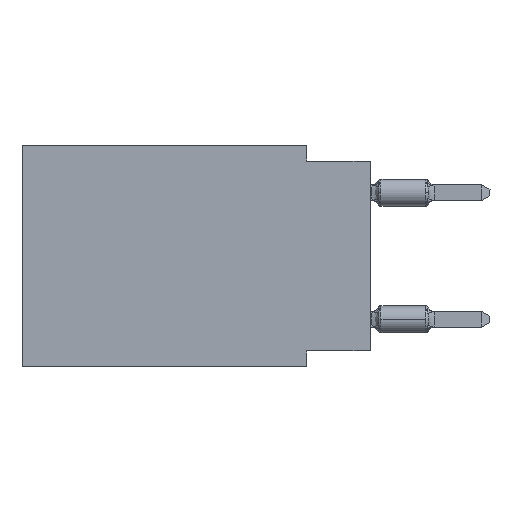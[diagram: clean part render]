
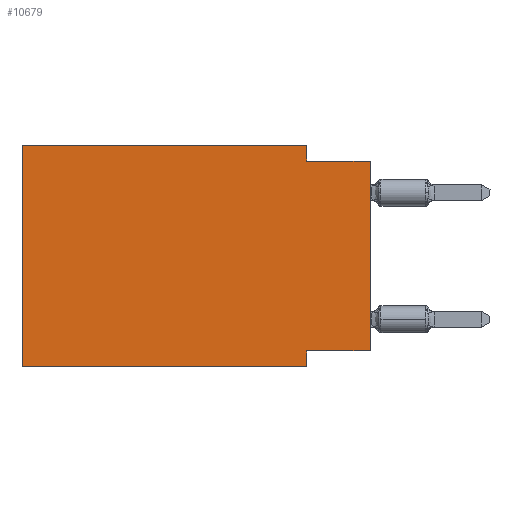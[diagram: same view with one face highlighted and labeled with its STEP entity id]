
A CAD part, left-side view. The second image highlights one B-rep face of the part: STEP entity #10679.
In plain terms, the highlighted planar face has unit normal (-1, 0, 0).
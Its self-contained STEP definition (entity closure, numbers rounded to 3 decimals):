
#524 = VERTEX_POINT ( 'NONE', #7464 ) ;
#616 = DIRECTION ( 'NONE',  ( 0., 0., -1. ) ) ;
#649 = VERTEX_POINT ( 'NONE', #11606 ) ;
#1061 = DIRECTION ( 'NONE',  ( 1., 0., 0. ) ) ;
#1350 = DIRECTION ( 'NONE',  ( 0., 0., -1. ) ) ;
#1417 = CARTESIAN_POINT ( 'NONE',  ( 0., 0., -0.635 ) ) ;
#1431 = VECTOR ( 'NONE', #5769, 1000. ) ;
#1520 = CARTESIAN_POINT ( 'NONE',  ( 0., 2.54, -8.89 ) ) ;
#1605 = VECTOR ( 'NONE', #3335, 1000. ) ;
#2075 = PLANE ( 'NONE',  #16275 ) ;
#2506 = VERTEX_POINT ( 'NONE', #13431 ) ;
#2578 = LINE ( 'NONE', #2665, #4321 ) ;
#2611 = CARTESIAN_POINT ( 'NONE',  ( 0., 2.54, -8.255 ) ) ;
#2660 = VECTOR ( 'NONE', #3162, 1000. ) ;
#2665 = CARTESIAN_POINT ( 'NONE',  ( 0., 13.97, 0. ) ) ;
#2909 = LINE ( 'NONE', #3078, #16213 ) ;
#2989 = EDGE_CURVE ( 'NONE', #14532, #4736, #7956, .T. ) ;
#3078 = CARTESIAN_POINT ( 'NONE',  ( 0., 2.54, 0. ) ) ;
#3086 = CARTESIAN_POINT ( 'NONE',  ( 0., 0., 0. ) ) ;
#3162 = DIRECTION ( 'NONE',  ( 0., 0., 1. ) ) ;
#3335 = DIRECTION ( 'NONE',  ( 0., -1., 0. ) ) ;
#3425 = VERTEX_POINT ( 'NONE', #1417 ) ;
#3804 = EDGE_CURVE ( 'NONE', #2506, #524, #2578, .T. ) ;
#3997 = EDGE_CURVE ( 'NONE', #8970, #649, #2909, .T. ) ;
#4321 = VECTOR ( 'NONE', #10536, 1000. ) ;
#4567 = ORIENTED_EDGE ( 'NONE', *, *, #10403, .F. ) ;
#4736 = VERTEX_POINT ( 'NONE', #14694 ) ;
#4797 = VECTOR ( 'NONE', #9881, 1000. ) ;
#5769 = DIRECTION ( 'NONE',  ( 0., -1., 0. ) ) ;
#5846 = ORIENTED_EDGE ( 'NONE', *, *, #11461, .F. ) ;
#6208 = CARTESIAN_POINT ( 'NONE',  ( 0., 0., -8.255 ) ) ;
#6268 = EDGE_CURVE ( 'NONE', #8893, #3425, #14682, .T. ) ;
#6305 = EDGE_CURVE ( 'NONE', #2506, #4736, #8497, .T. ) ;
#6626 = EDGE_LOOP ( 'NONE', ( #12194, #4567, #14651, #5846, #14333, #8191, #10826, #11144 ) ) ;
#6943 = DIRECTION ( 'NONE',  ( 0., -1., 0. ) ) ;
#7177 = LINE ( 'NONE', #10991, #4797 ) ;
#7240 = DIRECTION ( 'NONE',  ( 0., 0., -1. ) ) ;
#7464 = CARTESIAN_POINT ( 'NONE',  ( 0., 13.97, 0. ) ) ;
#7846 = VECTOR ( 'NONE', #1350, 1000. ) ;
#7956 = LINE ( 'NONE', #1520, #7846 ) ;
#8191 = ORIENTED_EDGE ( 'NONE', *, *, #6305, .T. ) ;
#8497 = LINE ( 'NONE', #12391, #1605 ) ;
#8893 = VERTEX_POINT ( 'NONE', #6208 ) ;
#8970 = VERTEX_POINT ( 'NONE', #15179 ) ;
#9487 = LINE ( 'NONE', #10760, #14908 ) ;
#9857 = CARTESIAN_POINT ( 'NONE',  ( 0., 13.97, 0. ) ) ;
#9881 = DIRECTION ( 'NONE',  ( 0., 1., 0. ) ) ;
#10403 = EDGE_CURVE ( 'NONE', #649, #3425, #9487, .T. ) ;
#10536 = DIRECTION ( 'NONE',  ( 0., 0., 1. ) ) ;
#10679 = ADVANCED_FACE ( 'NONE', ( #15207 ), #2075, .F. ) ;
#10760 = CARTESIAN_POINT ( 'NONE',  ( 0., 0., -0.635 ) ) ;
#10826 = ORIENTED_EDGE ( 'NONE', *, *, #2989, .F. ) ;
#10991 = CARTESIAN_POINT ( 'NONE',  ( 0., 0., -8.255 ) ) ;
#11144 = ORIENTED_EDGE ( 'NONE', *, *, #14564, .F. ) ;
#11461 = EDGE_CURVE ( 'NONE', #524, #8970, #14737, .T. ) ;
#11606 = CARTESIAN_POINT ( 'NONE',  ( 0., 2.54, -0.635 ) ) ;
#12194 = ORIENTED_EDGE ( 'NONE', *, *, #6268, .T. ) ;
#12391 = CARTESIAN_POINT ( 'NONE',  ( 0., 13.97, -8.89 ) ) ;
#13431 = CARTESIAN_POINT ( 'NONE',  ( 0., 13.97, -8.89 ) ) ;
#14333 = ORIENTED_EDGE ( 'NONE', *, *, #3804, .F. ) ;
#14532 = VERTEX_POINT ( 'NONE', #2611 ) ;
#14564 = EDGE_CURVE ( 'NONE', #8893, #14532, #7177, .T. ) ;
#14651 = ORIENTED_EDGE ( 'NONE', *, *, #3997, .F. ) ;
#14682 = LINE ( 'NONE', #3086, #2660 ) ;
#14694 = CARTESIAN_POINT ( 'NONE',  ( 0., 2.54, -8.89 ) ) ;
#14737 = LINE ( 'NONE', #14991, #1431 ) ;
#14908 = VECTOR ( 'NONE', #6943, 1000. ) ;
#14991 = CARTESIAN_POINT ( 'NONE',  ( 0., 13.97, 0. ) ) ;
#15179 = CARTESIAN_POINT ( 'NONE',  ( 0., 2.54, 0. ) ) ;
#15207 = FACE_OUTER_BOUND ( 'NONE', #6626, .T. ) ;
#16213 = VECTOR ( 'NONE', #616, 1000. ) ;
#16275 = AXIS2_PLACEMENT_3D ( 'NONE', #9857, #1061, #7240 ) ;
